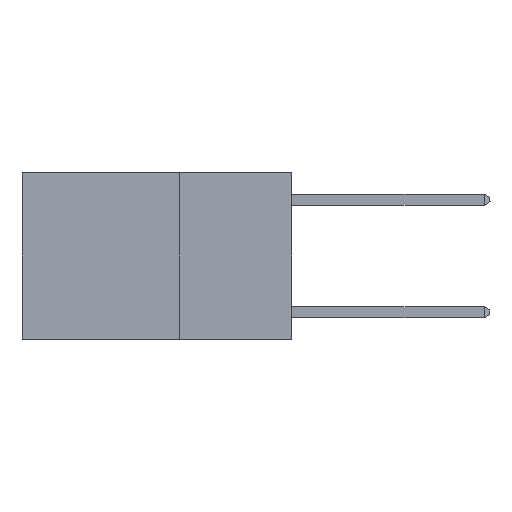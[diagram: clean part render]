
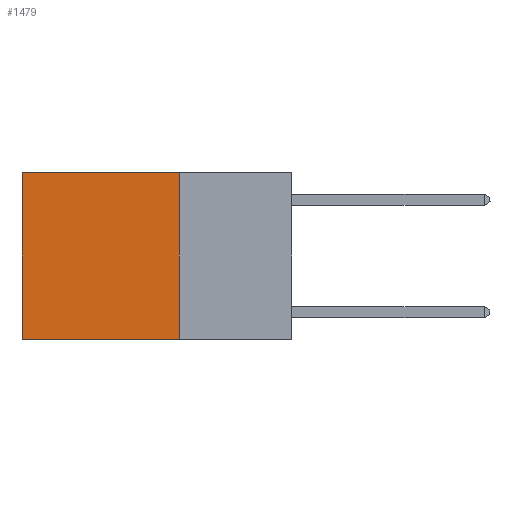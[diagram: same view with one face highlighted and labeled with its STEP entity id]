
A CAD part, left-side view. The second image highlights one B-rep face of the part: STEP entity #1479.
In plain terms, the highlighted planar face has unit normal (-1, 0, 0).
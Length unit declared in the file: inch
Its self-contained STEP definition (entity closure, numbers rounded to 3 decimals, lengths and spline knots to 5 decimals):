
#47 = ORIENTED_EDGE ( 'NONE', *, *, #2910, .F. ) ;
#211 = CARTESIAN_POINT ( 'NONE',  ( 0.2625, 0.25, 0. ) ) ;
#294 = CARTESIAN_POINT ( 'NONE',  ( 0.2625, 0.6, -0.37 ) ) ;
#357 = VECTOR ( 'NONE', #1315, 39.37008 ) ;
#511 = EDGE_CURVE ( 'NONE', #5574, #7029, #3574, .T. ) ;
#753 = CARTESIAN_POINT ( 'NONE',  ( 0.2625, 0.6, 0. ) ) ;
#931 = ORIENTED_EDGE ( 'NONE', *, *, #2087, .T. ) ;
#1012 = CARTESIAN_POINT ( 'NONE',  ( 0.2625, 0.25, 0. ) ) ;
#1315 = DIRECTION ( 'NONE',  ( 0., 1., 0. ) ) ;
#1435 = EDGE_CURVE ( 'NONE', #5574, #5749, #6105, .T. ) ;
#1479 = ADVANCED_FACE ( 'NONE', ( #3771 ), #7829, .F. ) ;
#1856 = EDGE_LOOP ( 'NONE', ( #931, #47, #1933, #6326 ) ) ;
#1933 = ORIENTED_EDGE ( 'NONE', *, *, #511, .F. ) ;
#2087 = EDGE_CURVE ( 'NONE', #5749, #3145, #7158, .T. ) ;
#2910 = EDGE_CURVE ( 'NONE', #7029, #3145, #3937, .T. ) ;
#3145 = VERTEX_POINT ( 'NONE', #294 ) ;
#3574 = LINE ( 'NONE', #7713, #3795 ) ;
#3771 = FACE_OUTER_BOUND ( 'NONE', #1856, .T. ) ;
#3795 = VECTOR ( 'NONE', #8352, 39.37008 ) ;
#3937 = LINE ( 'NONE', #5742, #7451 ) ;
#4060 = CARTESIAN_POINT ( 'NONE',  ( 0.2625, 0.25, -0.37 ) ) ;
#5255 = VECTOR ( 'NONE', #7855, 39.37008 ) ;
#5574 = VERTEX_POINT ( 'NONE', #211 ) ;
#5742 = CARTESIAN_POINT ( 'NONE',  ( 0.2625, 0.25, -0.37 ) ) ;
#5749 = VERTEX_POINT ( 'NONE', #7453 ) ;
#6105 = LINE ( 'NONE', #1012, #357 ) ;
#6326 = ORIENTED_EDGE ( 'NONE', *, *, #1435, .T. ) ;
#6468 = DIRECTION ( 'NONE',  ( 0., 1., 0. ) ) ;
#7029 = VERTEX_POINT ( 'NONE', #4060 ) ;
#7158 = LINE ( 'NONE', #753, #5255 ) ;
#7378 = AXIS2_PLACEMENT_3D ( 'NONE', #8152, #7820, #7775 ) ;
#7451 = VECTOR ( 'NONE', #6468, 39.37008 ) ;
#7453 = CARTESIAN_POINT ( 'NONE',  ( 0.2625, 0.6, 0. ) ) ;
#7713 = CARTESIAN_POINT ( 'NONE',  ( 0.2625, 0.25, 0. ) ) ;
#7775 = DIRECTION ( 'NONE',  ( 0., 0., -1. ) ) ;
#7820 = DIRECTION ( 'NONE',  ( 1., 0., 0. ) ) ;
#7829 = PLANE ( 'NONE',  #7378 ) ;
#7855 = DIRECTION ( 'NONE',  ( 0., 0., -1. ) ) ;
#8152 = CARTESIAN_POINT ( 'NONE',  ( 0.2625, 0.25, 0. ) ) ;
#8352 = DIRECTION ( 'NONE',  ( 0., 0., -1. ) ) ;
